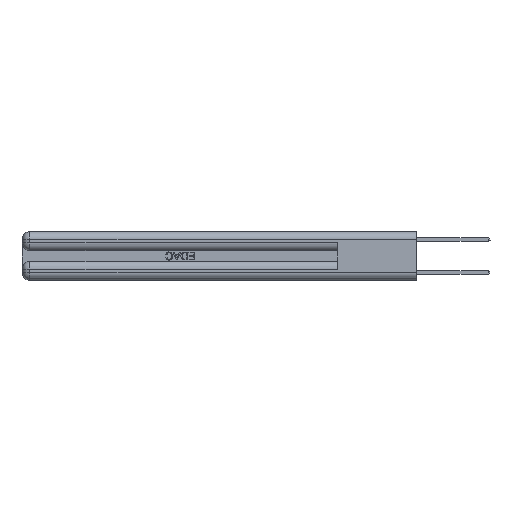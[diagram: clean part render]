
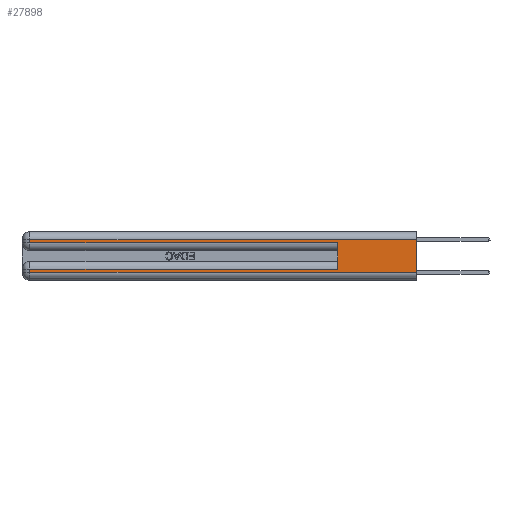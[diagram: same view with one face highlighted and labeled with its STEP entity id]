
A CAD part, left-side view. The second image highlights one B-rep face of the part: STEP entity #27898.
In plain terms, the highlighted planar face has unit normal (-1, 0, 0).
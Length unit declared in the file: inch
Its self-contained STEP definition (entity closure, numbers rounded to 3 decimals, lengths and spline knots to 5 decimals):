
#611 = DIRECTION ( 'NONE',  ( 0., 1., 0. ) ) ;
#1366 = CARTESIAN_POINT ( 'NONE',  ( 0., 2.94, 0.06 ) ) ;
#1382 = VERTEX_POINT ( 'NONE', #12227 ) ;
#1552 = EDGE_CURVE ( 'NONE', #19825, #1382, #14962, .T. ) ;
#2369 = CARTESIAN_POINT ( 'NONE',  ( 0., 2.94, 0.37 ) ) ;
#2699 = DIRECTION ( 'NONE',  ( 0., -1., 0. ) ) ;
#3128 = EDGE_CURVE ( 'NONE', #28425, #17028, #11921, .T. ) ;
#3336 = DIRECTION ( 'NONE',  ( 0., 0., -1. ) ) ;
#3589 = EDGE_CURVE ( 'NONE', #28425, #1382, #32960, .T. ) ;
#3661 = CARTESIAN_POINT ( 'NONE',  ( 0., 0.6, 0.085 ) ) ;
#4647 = ORIENTED_EDGE ( 'NONE', *, *, #21891, .T. ) ;
#4801 = CARTESIAN_POINT ( 'NONE',  ( 0., 0.6, 0.145 ) ) ;
#4941 = CARTESIAN_POINT ( 'NONE',  ( 0., 2.94, 0.085 ) ) ;
#6275 = EDGE_LOOP ( 'NONE', ( #16128, #18501, #4647, #15768, #11811, #7497, #14366, #29626 ) ) ;
#6798 = CARTESIAN_POINT ( 'NONE',  ( 0., 0., 0.37 ) ) ;
#7380 = VERTEX_POINT ( 'NONE', #21622 ) ;
#7497 = ORIENTED_EDGE ( 'NONE', *, *, #33990, .T. ) ;
#7863 = VECTOR ( 'NONE', #17616, 39.37008 ) ;
#8120 = VECTOR ( 'NONE', #33664, 39.37008 ) ;
#8150 = VERTEX_POINT ( 'NONE', #4941 ) ;
#8890 = VERTEX_POINT ( 'NONE', #3661 ) ;
#9350 = VERTEX_POINT ( 'NONE', #21879 ) ;
#11065 = PLANE ( 'NONE',  #28462 ) ;
#11197 = DIRECTION ( 'NONE',  ( 1., 0., 0. ) ) ;
#11811 = ORIENTED_EDGE ( 'NONE', *, *, #28550, .F. ) ;
#11915 = CARTESIAN_POINT ( 'NONE',  ( 0., 0., 0.37 ) ) ;
#11921 = LINE ( 'NONE', #14246, #33403 ) ;
#12227 = CARTESIAN_POINT ( 'NONE',  ( 0., 0., 0.06 ) ) ;
#12663 = DIRECTION ( 'NONE',  ( 0., 1., 0. ) ) ;
#13389 = FACE_OUTER_BOUND ( 'NONE', #6275, .T. ) ;
#14246 = CARTESIAN_POINT ( 'NONE',  ( 0., 0., 0.31 ) ) ;
#14366 = ORIENTED_EDGE ( 'NONE', *, *, #32084, .T. ) ;
#14962 = LINE ( 'NONE', #24490, #7863 ) ;
#15768 = ORIENTED_EDGE ( 'NONE', *, *, #30272, .T. ) ;
#15835 = CARTESIAN_POINT ( 'NONE',  ( 0., 0., 0.31 ) ) ;
#16128 = ORIENTED_EDGE ( 'NONE', *, *, #3589, .F. ) ;
#16443 = VECTOR ( 'NONE', #12663, 39.37008 ) ;
#16829 = CARTESIAN_POINT ( 'NONE',  ( 0., 2.94, 0.31 ) ) ;
#17028 = VERTEX_POINT ( 'NONE', #16829 ) ;
#17616 = DIRECTION ( 'NONE',  ( 0., -1., 0. ) ) ;
#18501 = ORIENTED_EDGE ( 'NONE', *, *, #3128, .T. ) ;
#19533 = VECTOR ( 'NONE', #23035, 39.37008 ) ;
#19825 = VERTEX_POINT ( 'NONE', #1366 ) ;
#20828 = DIRECTION ( 'NONE',  ( 0., 0., -1. ) ) ;
#21622 = CARTESIAN_POINT ( 'NONE',  ( 0., 2.94, 0.285 ) ) ;
#21879 = CARTESIAN_POINT ( 'NONE',  ( 0., 0.6, 0.285 ) ) ;
#21891 = EDGE_CURVE ( 'NONE', #17028, #7380, #26584, .T. ) ;
#23035 = DIRECTION ( 'NONE',  ( 0., 0., -1. ) ) ;
#23513 = LINE ( 'NONE', #27921, #16443 ) ;
#23741 = DIRECTION ( 'NONE',  ( 0., 0., 1. ) ) ;
#24490 = CARTESIAN_POINT ( 'NONE',  ( 0., 0., 0.06 ) ) ;
#26350 = CARTESIAN_POINT ( 'NONE',  ( 0., 0., 0.285 ) ) ;
#26584 = LINE ( 'NONE', #2369, #33163 ) ;
#27898 = ADVANCED_FACE ( 'NONE', ( #13389 ), #11065, .F. ) ;
#27921 = CARTESIAN_POINT ( 'NONE',  ( 0., 0., 0.085 ) ) ;
#28425 = VERTEX_POINT ( 'NONE', #15835 ) ;
#28462 = AXIS2_PLACEMENT_3D ( 'NONE', #11915, #11197, #3336 ) ;
#28550 = EDGE_CURVE ( 'NONE', #8890, #9350, #30503, .T. ) ;
#28730 = VECTOR ( 'NONE', #2699, 39.37008 ) ;
#29626 = ORIENTED_EDGE ( 'NONE', *, *, #1552, .T. ) ;
#29856 = LINE ( 'NONE', #33822, #19533 ) ;
#30272 = EDGE_CURVE ( 'NONE', #7380, #9350, #34073, .T. ) ;
#30503 = LINE ( 'NONE', #4801, #31317 ) ;
#31317 = VECTOR ( 'NONE', #23741, 39.37008 ) ;
#32084 = EDGE_CURVE ( 'NONE', #8150, #19825, #29856, .T. ) ;
#32960 = LINE ( 'NONE', #6798, #8120 ) ;
#33163 = VECTOR ( 'NONE', #20828, 39.37008 ) ;
#33403 = VECTOR ( 'NONE', #611, 39.37008 ) ;
#33664 = DIRECTION ( 'NONE',  ( 0., 0., -1. ) ) ;
#33822 = CARTESIAN_POINT ( 'NONE',  ( 0., 2.94, 0.37 ) ) ;
#33990 = EDGE_CURVE ( 'NONE', #8890, #8150, #23513, .T. ) ;
#34073 = LINE ( 'NONE', #26350, #28730 ) ;
